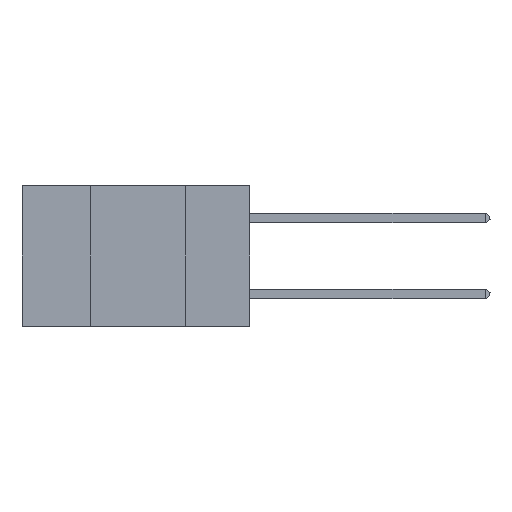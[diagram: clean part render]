
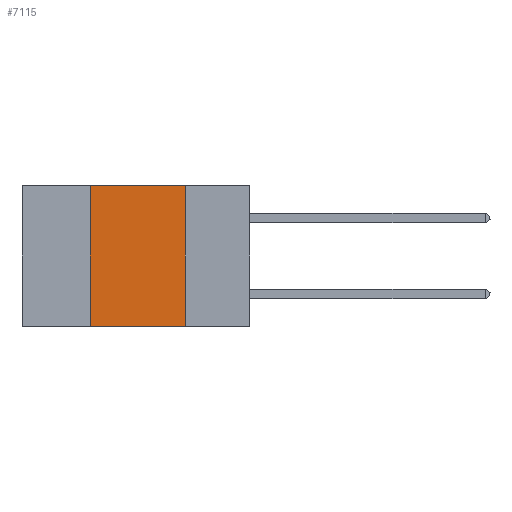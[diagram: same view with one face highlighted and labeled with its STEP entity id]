
A CAD part, left-side view. The second image highlights one B-rep face of the part: STEP entity #7115.
In plain terms, the highlighted planar face has unit normal (-1, 0, 0).
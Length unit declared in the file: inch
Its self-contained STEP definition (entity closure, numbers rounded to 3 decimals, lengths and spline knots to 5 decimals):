
#264 = CARTESIAN_POINT ( 'NONE',  ( 0., 0.17, -0.37 ) ) ;
#464 = CARTESIAN_POINT ( 'NONE',  ( 0., 0.42, -0.37 ) ) ;
#729 = EDGE_CURVE ( 'NONE', #17125, #18948, #4344, .T. ) ;
#1580 = CARTESIAN_POINT ( 'NONE',  ( 0., 0.42, 0. ) ) ;
#1732 = LINE ( 'NONE', #20846, #12299 ) ;
#3198 = ORIENTED_EDGE ( 'NONE', *, *, #15529, .F. ) ;
#3364 = DIRECTION ( 'NONE',  ( 0., -1., 0. ) ) ;
#3879 = FACE_OUTER_BOUND ( 'NONE', #16252, .T. ) ;
#4195 = LINE ( 'NONE', #13280, #9830 ) ;
#4220 = CARTESIAN_POINT ( 'NONE',  ( 0., 0.42, 0. ) ) ;
#4344 = LINE ( 'NONE', #1580, #8105 ) ;
#4508 = PLANE ( 'NONE',  #10895 ) ;
#4522 = LINE ( 'NONE', #6977, #21066 ) ;
#4580 = DIRECTION ( 'NONE',  ( 1., 0., 0. ) ) ;
#4941 = ORIENTED_EDGE ( 'NONE', *, *, #729, .F. ) ;
#5582 = DIRECTION ( 'NONE',  ( 0., 0., 1. ) ) ;
#6977 = CARTESIAN_POINT ( 'NONE',  ( 0., 0.6, -0.37 ) ) ;
#7115 = ADVANCED_FACE ( 'NONE', ( #3879 ), #4508, .F. ) ;
#8105 = VECTOR ( 'NONE', #5582, 39.37008 ) ;
#8206 = ORIENTED_EDGE ( 'NONE', *, *, #15447, .T. ) ;
#9830 = VECTOR ( 'NONE', #3364, 39.37008 ) ;
#10389 = CARTESIAN_POINT ( 'NONE',  ( 0., 0.17, 0. ) ) ;
#10895 = AXIS2_PLACEMENT_3D ( 'NONE', #22382, #4580, #14503 ) ;
#11086 = DIRECTION ( 'NONE',  ( 0., 0., -1. ) ) ;
#12299 = VECTOR ( 'NONE', #11086, 39.37008 ) ;
#13280 = CARTESIAN_POINT ( 'NONE',  ( 0., 0.6, 0. ) ) ;
#14172 = VERTEX_POINT ( 'NONE', #10389 ) ;
#14503 = DIRECTION ( 'NONE',  ( 0., 0., -1. ) ) ;
#15447 = EDGE_CURVE ( 'NONE', #17125, #16996, #4522, .T. ) ;
#15529 = EDGE_CURVE ( 'NONE', #14172, #16996, #1732, .T. ) ;
#16252 = EDGE_LOOP ( 'NONE', ( #3198, #24731, #4941, #8206 ) ) ;
#16996 = VERTEX_POINT ( 'NONE', #264 ) ;
#17125 = VERTEX_POINT ( 'NONE', #464 ) ;
#18948 = VERTEX_POINT ( 'NONE', #4220 ) ;
#19060 = EDGE_CURVE ( 'NONE', #18948, #14172, #4195, .T. ) ;
#20846 = CARTESIAN_POINT ( 'NONE',  ( 0., 0.17, 0. ) ) ;
#21066 = VECTOR ( 'NONE', #21182, 39.37008 ) ;
#21182 = DIRECTION ( 'NONE',  ( 0., -1., 0. ) ) ;
#22382 = CARTESIAN_POINT ( 'NONE',  ( 0., 0.6, 0. ) ) ;
#24731 = ORIENTED_EDGE ( 'NONE', *, *, #19060, .F. ) ;
